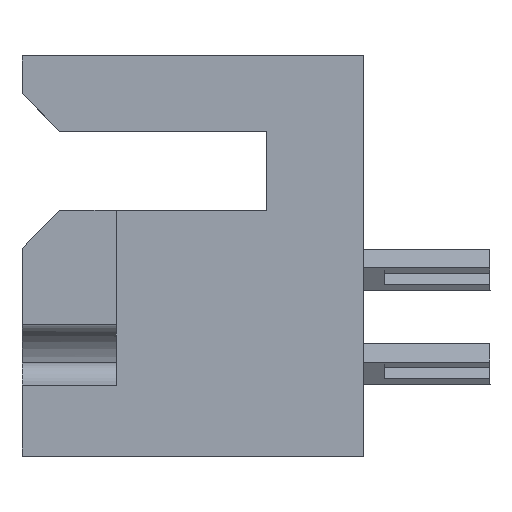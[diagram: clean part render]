
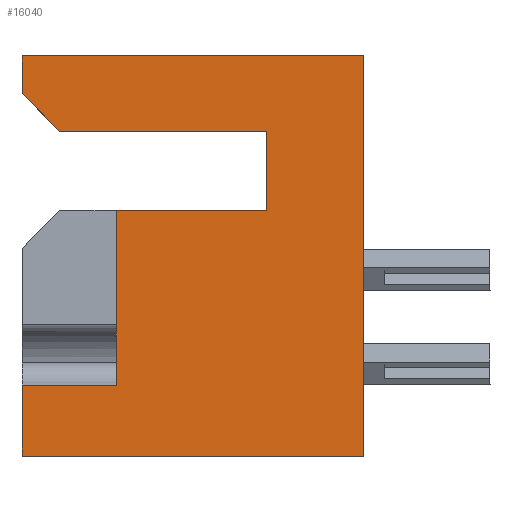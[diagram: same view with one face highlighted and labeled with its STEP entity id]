
A CAD part, left-side view. The second image highlights one B-rep face of the part: STEP entity #16040.
In plain terms, the highlighted planar face has unit normal (-1, 0, 0).
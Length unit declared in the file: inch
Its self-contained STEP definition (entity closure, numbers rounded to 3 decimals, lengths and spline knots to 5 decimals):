
#310 = VERTEX_POINT ( 'NONE', #3868 ) ;
#456 = VECTOR ( 'NONE', #8500, 39.37008 ) ;
#871 = CARTESIAN_POINT ( 'NONE',  ( 0., 0.328, -0.205 ) ) ;
#1003 = VERTEX_POINT ( 'NONE', #19327 ) ;
#1545 = VERTEX_POINT ( 'NONE', #24366 ) ;
#1784 = DIRECTION ( 'NONE',  ( 0., 1., 0. ) ) ;
#1829 = CARTESIAN_POINT ( 'NONE',  ( 0., 0.403, -0.1 ) ) ;
#1842 = CARTESIAN_POINT ( 'NONE',  ( 0., 0.128, -0.1 ) ) ;
#1970 = EDGE_CURVE ( 'NONE', #25563, #23127, #3062, .T. ) ;
#2292 = ORIENTED_EDGE ( 'NONE', *, *, #19497, .T. ) ;
#2452 = CARTESIAN_POINT ( 'NONE',  ( 0., 0.453, 0. ) ) ;
#2534 = VECTOR ( 'NONE', #23929, 39.37008 ) ;
#3062 = LINE ( 'NONE', #22848, #24751 ) ;
#3092 = EDGE_CURVE ( 'NONE', #23301, #23127, #8680, .T. ) ;
#3245 = DIRECTION ( 'NONE',  ( 0., 0., 1. ) ) ;
#3562 = EDGE_CURVE ( 'NONE', #22932, #1003, #4727, .T. ) ;
#3635 = EDGE_LOOP ( 'NONE', ( #24438, #3652, #14443, #2292, #6119, #12577, #6514, #6505, #24437, #11041, #15339 ) ) ;
#3652 = ORIENTED_EDGE ( 'NONE', *, *, #5263, .F. ) ;
#3868 = CARTESIAN_POINT ( 'NONE',  ( 0., 0.328, -0.437 ) ) ;
#4223 = LINE ( 'NONE', #871, #23303 ) ;
#4727 = LINE ( 'NONE', #15528, #20820 ) ;
#4759 = DIRECTION ( 'NONE',  ( 1., 0., 0. ) ) ;
#5148 = VECTOR ( 'NONE', #3245, 39.37008 ) ;
#5263 = EDGE_CURVE ( 'NONE', #22932, #9921, #10857, .T. ) ;
#5560 = DIRECTION ( 'NONE',  ( 0., -0.707, -0.707 ) ) ;
#5633 = EDGE_CURVE ( 'NONE', #310, #9921, #7225, .T. ) ;
#6119 = ORIENTED_EDGE ( 'NONE', *, *, #20295, .F. ) ;
#6505 = ORIENTED_EDGE ( 'NONE', *, *, #1970, .F. ) ;
#6514 = ORIENTED_EDGE ( 'NONE', *, *, #3092, .T. ) ;
#7036 = CARTESIAN_POINT ( 'NONE',  ( 0., 0.128, -0.205 ) ) ;
#7225 = LINE ( 'NONE', #25009, #25980 ) ;
#8037 = EDGE_CURVE ( 'NONE', #310, #25351, #4223, .T. ) ;
#8500 = DIRECTION ( 'NONE',  ( 0., -1., 0. ) ) ;
#8680 = LINE ( 'NONE', #18130, #14578 ) ;
#8716 = LINE ( 'NONE', #23140, #456 ) ;
#9921 = VERTEX_POINT ( 'NONE', #23523 ) ;
#10374 = DIRECTION ( 'NONE',  ( 0., 1., 0. ) ) ;
#10857 = LINE ( 'NONE', #25376, #18701 ) ;
#10880 = VERTEX_POINT ( 'NONE', #13879 ) ;
#11041 = ORIENTED_EDGE ( 'NONE', *, *, #11313, .T. ) ;
#11255 = DIRECTION ( 'NONE',  ( 0., 0., 1. ) ) ;
#11302 = VECTOR ( 'NONE', #19252, 39.37008 ) ;
#11313 = EDGE_CURVE ( 'NONE', #23158, #25351, #18961, .T. ) ;
#11854 = CARTESIAN_POINT ( 'NONE',  ( 0., 0.328, -0.205 ) ) ;
#12241 = AXIS2_PLACEMENT_3D ( 'NONE', #19693, #4759, #25775 ) ;
#12577 = ORIENTED_EDGE ( 'NONE', *, *, #27008, .F. ) ;
#12965 = DIRECTION ( 'NONE',  ( 0., 0., 1. ) ) ;
#13879 = CARTESIAN_POINT ( 'NONE',  ( 0., 0.453, 0. ) ) ;
#14443 = ORIENTED_EDGE ( 'NONE', *, *, #3562, .T. ) ;
#14578 = VECTOR ( 'NONE', #5560, 39.37008 ) ;
#15339 = ORIENTED_EDGE ( 'NONE', *, *, #8037, .F. ) ;
#15528 = CARTESIAN_POINT ( 'NONE',  ( 0., 0.453, -0.531 ) ) ;
#15810 = CARTESIAN_POINT ( 'NONE',  ( 0., 0., 0. ) ) ;
#16040 = ADVANCED_FACE ( 'NONE', ( #18214 ), #26041, .F. ) ;
#17203 = DIRECTION ( 'NONE',  ( 0., 0., 1. ) ) ;
#17607 = LINE ( 'NONE', #15810, #5148 ) ;
#17642 = CARTESIAN_POINT ( 'NONE',  ( 0., 0.453, -0.531 ) ) ;
#17821 = DIRECTION ( 'NONE',  ( 0., -1., 0. ) ) ;
#18130 = CARTESIAN_POINT ( 'NONE',  ( 0., 0.403, -0.1 ) ) ;
#18214 = FACE_OUTER_BOUND ( 'NONE', #3635, .T. ) ;
#18701 = VECTOR ( 'NONE', #12965, 39.37008 ) ;
#18961 = LINE ( 'NONE', #7036, #2534 ) ;
#19252 = DIRECTION ( 'NONE',  ( 0., 0., 1. ) ) ;
#19327 = CARTESIAN_POINT ( 'NONE',  ( 0., 0., -0.531 ) ) ;
#19497 = EDGE_CURVE ( 'NONE', #1003, #1545, #17607, .T. ) ;
#19693 = CARTESIAN_POINT ( 'NONE',  ( 0., 0.453, 0. ) ) ;
#20199 = LINE ( 'NONE', #2452, #11302 ) ;
#20295 = EDGE_CURVE ( 'NONE', #10880, #1545, #8716, .T. ) ;
#20335 = LINE ( 'NONE', #25402, #25268 ) ;
#20820 = VECTOR ( 'NONE', #17821, 39.37008 ) ;
#22848 = CARTESIAN_POINT ( 'NONE',  ( 0., 0.128, -0.1 ) ) ;
#22932 = VERTEX_POINT ( 'NONE', #17642 ) ;
#23127 = VERTEX_POINT ( 'NONE', #1829 ) ;
#23140 = CARTESIAN_POINT ( 'NONE',  ( 0., 0.453, 0. ) ) ;
#23158 = VERTEX_POINT ( 'NONE', #24729 ) ;
#23301 = VERTEX_POINT ( 'NONE', #25729 ) ;
#23303 = VECTOR ( 'NONE', #11255, 39.37008 ) ;
#23523 = CARTESIAN_POINT ( 'NONE',  ( 0., 0.453, -0.437 ) ) ;
#23929 = DIRECTION ( 'NONE',  ( 0., 1., 0. ) ) ;
#24366 = CARTESIAN_POINT ( 'NONE',  ( 0., 0., 0. ) ) ;
#24437 = ORIENTED_EDGE ( 'NONE', *, *, #24496, .F. ) ;
#24438 = ORIENTED_EDGE ( 'NONE', *, *, #5633, .T. ) ;
#24496 = EDGE_CURVE ( 'NONE', #23158, #25563, #20335, .T. ) ;
#24729 = CARTESIAN_POINT ( 'NONE',  ( 0., 0.128, -0.205 ) ) ;
#24751 = VECTOR ( 'NONE', #1784, 39.37008 ) ;
#25009 = CARTESIAN_POINT ( 'NONE',  ( 0., 0.328, -0.437 ) ) ;
#25268 = VECTOR ( 'NONE', #17203, 39.37008 ) ;
#25351 = VERTEX_POINT ( 'NONE', #11854 ) ;
#25376 = CARTESIAN_POINT ( 'NONE',  ( 0., 0.453, 0. ) ) ;
#25402 = CARTESIAN_POINT ( 'NONE',  ( 0., 0.128, -0.1 ) ) ;
#25563 = VERTEX_POINT ( 'NONE', #1842 ) ;
#25729 = CARTESIAN_POINT ( 'NONE',  ( 0., 0.453, -0.05 ) ) ;
#25775 = DIRECTION ( 'NONE',  ( 0., 0., -1. ) ) ;
#25980 = VECTOR ( 'NONE', #10374, 39.37008 ) ;
#26041 = PLANE ( 'NONE',  #12241 ) ;
#27008 = EDGE_CURVE ( 'NONE', #23301, #10880, #20199, .T. ) ;
